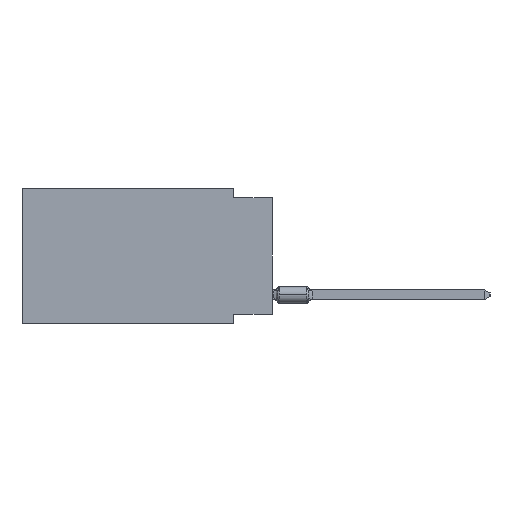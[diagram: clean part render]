
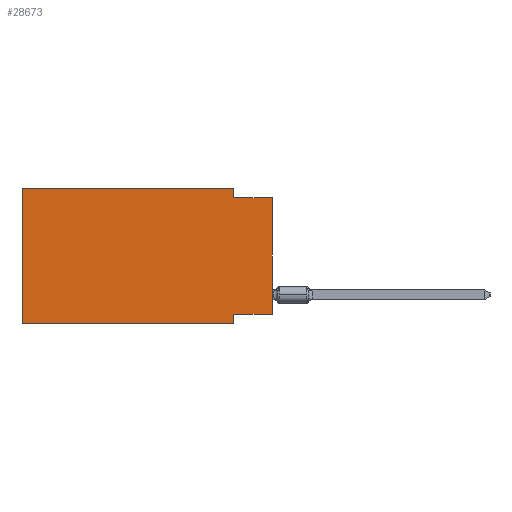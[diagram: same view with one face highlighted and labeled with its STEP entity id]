
A CAD part, left-side view. The second image highlights one B-rep face of the part: STEP entity #28673.
In plain terms, the highlighted planar face has unit normal (-1, 0, 0).
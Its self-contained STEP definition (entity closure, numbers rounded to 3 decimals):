
#621 = CARTESIAN_POINT ( 'NONE',  ( 0., 2.54, 0. ) ) ;
#1724 = CARTESIAN_POINT ( 'NONE',  ( 0., 16.383, 0. ) ) ;
#1997 = VERTEX_POINT ( 'NONE', #34719 ) ;
#2350 = CARTESIAN_POINT ( 'NONE',  ( 0., 2.54, -0.635 ) ) ;
#2401 = VERTEX_POINT ( 'NONE', #2350 ) ;
#2510 = LINE ( 'NONE', #22975, #33744 ) ;
#3244 = LINE ( 'NONE', #30289, #17127 ) ;
#3924 = DIRECTION ( 'NONE',  ( 1., 0., 0. ) ) ;
#4807 = DIRECTION ( 'NONE',  ( 0., -1., 0. ) ) ;
#5142 = DIRECTION ( 'NONE',  ( 0., 0., 1. ) ) ;
#5412 = EDGE_CURVE ( 'NONE', #1997, #13494, #7474, .T. ) ;
#5417 = LINE ( 'NONE', #17210, #12243 ) ;
#6243 = DIRECTION ( 'NONE',  ( 0., 0., 1. ) ) ;
#6909 = AXIS2_PLACEMENT_3D ( 'NONE', #1724, #3924, #36006 ) ;
#7155 = VERTEX_POINT ( 'NONE', #36695 ) ;
#7253 = VECTOR ( 'NONE', #30184, 1000. ) ;
#7415 = EDGE_CURVE ( 'NONE', #36039, #11830, #3244, .T. ) ;
#7474 = LINE ( 'NONE', #13825, #30679 ) ;
#9144 = ORIENTED_EDGE ( 'NONE', *, *, #37818, .F. ) ;
#9667 = DIRECTION ( 'NONE',  ( 0., -1., 0. ) ) ;
#10720 = ORIENTED_EDGE ( 'NONE', *, *, #34681, .F. ) ;
#11262 = ORIENTED_EDGE ( 'NONE', *, *, #5412, .F. ) ;
#11358 = CARTESIAN_POINT ( 'NONE',  ( 0., 2.54, -8.89 ) ) ;
#11830 = VERTEX_POINT ( 'NONE', #28657 ) ;
#12243 = VECTOR ( 'NONE', #29004, 1000. ) ;
#12560 = CARTESIAN_POINT ( 'NONE',  ( 0., 0., -0.635 ) ) ;
#13185 = ORIENTED_EDGE ( 'NONE', *, *, #7415, .F. ) ;
#13472 = VECTOR ( 'NONE', #9667, 1000. ) ;
#13494 = VERTEX_POINT ( 'NONE', #26283 ) ;
#13825 = CARTESIAN_POINT ( 'NONE',  ( 0., 16.383, 0. ) ) ;
#14239 = EDGE_LOOP ( 'NONE', ( #15783, #9144, #32002, #10720, #11262, #23244, #32824, #13185 ) ) ;
#14286 = DIRECTION ( 'NONE',  ( 0., -1., 0. ) ) ;
#14896 = EDGE_CURVE ( 'NONE', #26626, #2401, #27091, .T. ) ;
#15599 = CARTESIAN_POINT ( 'NONE',  ( 0., 2.54, 0. ) ) ;
#15783 = ORIENTED_EDGE ( 'NONE', *, *, #31340, .T. ) ;
#17127 = VECTOR ( 'NONE', #32997, 1000. ) ;
#17210 = CARTESIAN_POINT ( 'NONE',  ( 0., 2.54, -8.89 ) ) ;
#18413 = FACE_OUTER_BOUND ( 'NONE', #14239, .T. ) ;
#20071 = EDGE_CURVE ( 'NONE', #1997, #36129, #2510, .T. ) ;
#20437 = CARTESIAN_POINT ( 'NONE',  ( 0., 0., -8.255 ) ) ;
#22975 = CARTESIAN_POINT ( 'NONE',  ( 0., 16.383, -8.89 ) ) ;
#23244 = ORIENTED_EDGE ( 'NONE', *, *, #20071, .T. ) ;
#25443 = EDGE_CURVE ( 'NONE', #11830, #36129, #5417, .T. ) ;
#26263 = VECTOR ( 'NONE', #4807, 1000. ) ;
#26283 = CARTESIAN_POINT ( 'NONE',  ( 0., 16.383, 0. ) ) ;
#26626 = VERTEX_POINT ( 'NONE', #15599 ) ;
#26904 = LINE ( 'NONE', #27101, #31113 ) ;
#27091 = LINE ( 'NONE', #621, #7253 ) ;
#27101 = CARTESIAN_POINT ( 'NONE',  ( 0., 0., 0. ) ) ;
#27495 = PLANE ( 'NONE',  #6909 ) ;
#27638 = LINE ( 'NONE', #12560, #13472 ) ;
#27818 = LINE ( 'NONE', #28180, #26263 ) ;
#28180 = CARTESIAN_POINT ( 'NONE',  ( 0., 16.383, 0. ) ) ;
#28657 = CARTESIAN_POINT ( 'NONE',  ( 0., 2.54, -8.255 ) ) ;
#28673 = ADVANCED_FACE ( 'NONE', ( #18413 ), #27495, .F. ) ;
#29004 = DIRECTION ( 'NONE',  ( 0., 0., -1. ) ) ;
#30184 = DIRECTION ( 'NONE',  ( 0., 0., -1. ) ) ;
#30289 = CARTESIAN_POINT ( 'NONE',  ( 0., 0., -8.255 ) ) ;
#30679 = VECTOR ( 'NONE', #5142, 1000. ) ;
#31113 = VECTOR ( 'NONE', #6243, 1000. ) ;
#31340 = EDGE_CURVE ( 'NONE', #36039, #7155, #26904, .T. ) ;
#32002 = ORIENTED_EDGE ( 'NONE', *, *, #14896, .F. ) ;
#32824 = ORIENTED_EDGE ( 'NONE', *, *, #25443, .F. ) ;
#32997 = DIRECTION ( 'NONE',  ( 0., 1., 0. ) ) ;
#33744 = VECTOR ( 'NONE', #14286, 1000. ) ;
#34681 = EDGE_CURVE ( 'NONE', #13494, #26626, #27818, .T. ) ;
#34719 = CARTESIAN_POINT ( 'NONE',  ( 0., 16.383, -8.89 ) ) ;
#36006 = DIRECTION ( 'NONE',  ( 0., 0., -1. ) ) ;
#36039 = VERTEX_POINT ( 'NONE', #20437 ) ;
#36129 = VERTEX_POINT ( 'NONE', #11358 ) ;
#36695 = CARTESIAN_POINT ( 'NONE',  ( 0., 0., -0.635 ) ) ;
#37818 = EDGE_CURVE ( 'NONE', #2401, #7155, #27638, .T. ) ;
